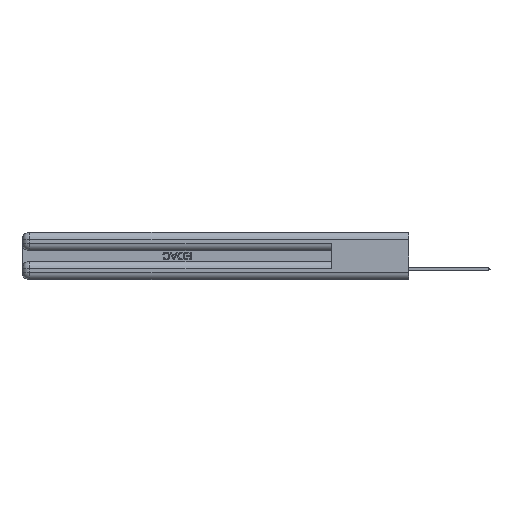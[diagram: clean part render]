
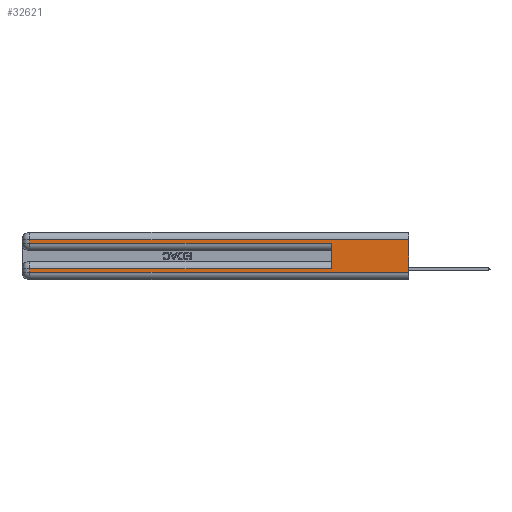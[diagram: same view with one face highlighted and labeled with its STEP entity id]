
A CAD part, left-side view. The second image highlights one B-rep face of the part: STEP entity #32621.
In plain terms, the highlighted planar face has unit normal (-1, 0, 0).
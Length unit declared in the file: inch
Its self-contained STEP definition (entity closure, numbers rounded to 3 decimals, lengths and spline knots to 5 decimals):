
#1006 = EDGE_CURVE ( 'NONE', #19458, #11600, #33406, .T. ) ;
#1236 = VECTOR ( 'NONE', #7126, 39.37008 ) ;
#3824 = CARTESIAN_POINT ( 'NONE',  ( 0., 0., 0.06 ) ) ;
#3852 = CARTESIAN_POINT ( 'NONE',  ( 0., 2.94, 0.06 ) ) ;
#3919 = VECTOR ( 'NONE', #11406, 39.37008 ) ;
#4619 = VECTOR ( 'NONE', #36373, 39.37008 ) ;
#5745 = VERTEX_POINT ( 'NONE', #46463 ) ;
#6093 = CARTESIAN_POINT ( 'NONE',  ( 0., 2.94, 0.31 ) ) ;
#6410 = LINE ( 'NONE', #38191, #3919 ) ;
#6543 = DIRECTION ( 'NONE',  ( 0., 1., 0. ) ) ;
#6690 = EDGE_CURVE ( 'NONE', #17661, #47163, #33459, .T. ) ;
#7126 = DIRECTION ( 'NONE',  ( 0., 1., 0. ) ) ;
#7585 = LINE ( 'NONE', #3824, #41613 ) ;
#8879 = CARTESIAN_POINT ( 'NONE',  ( 0., 2.94, 0.085 ) ) ;
#9315 = VERTEX_POINT ( 'NONE', #3852 ) ;
#9383 = ORIENTED_EDGE ( 'NONE', *, *, #12408, .T. ) ;
#11406 = DIRECTION ( 'NONE',  ( 0., -1., 0. ) ) ;
#11463 = CARTESIAN_POINT ( 'NONE',  ( 0., 0., 0.31 ) ) ;
#11600 = VERTEX_POINT ( 'NONE', #6093 ) ;
#12283 = ORIENTED_EDGE ( 'NONE', *, *, #15219, .T. ) ;
#12408 = EDGE_CURVE ( 'NONE', #11600, #37353, #27180, .T. ) ;
#15219 = EDGE_CURVE ( 'NONE', #9315, #5745, #7585, .T. ) ;
#16468 = LINE ( 'NONE', #27499, #38586 ) ;
#16790 = ORIENTED_EDGE ( 'NONE', *, *, #1006, .T. ) ;
#17089 = PLANE ( 'NONE',  #28386 ) ;
#17661 = VERTEX_POINT ( 'NONE', #50497 ) ;
#18962 = VECTOR ( 'NONE', #6543, 39.37008 ) ;
#19458 = VERTEX_POINT ( 'NONE', #26622 ) ;
#21163 = EDGE_CURVE ( 'NONE', #19458, #5745, #16468, .T. ) ;
#21610 = EDGE_CURVE ( 'NONE', #37353, #49317, #6410, .T. ) ;
#21665 = CARTESIAN_POINT ( 'NONE',  ( 0., 0., 0.37 ) ) ;
#22977 = ORIENTED_EDGE ( 'NONE', *, *, #21610, .T. ) ;
#23033 = DIRECTION ( 'NONE',  ( 0., 0., -1. ) ) ;
#24056 = EDGE_CURVE ( 'NONE', #17661, #49317, #38378, .T. ) ;
#25416 = DIRECTION ( 'NONE',  ( 0., 0., -1. ) ) ;
#26622 = CARTESIAN_POINT ( 'NONE',  ( 0., 0., 0.31 ) ) ;
#27152 = ORIENTED_EDGE ( 'NONE', *, *, #24056, .F. ) ;
#27180 = LINE ( 'NONE', #50384, #32761 ) ;
#27499 = CARTESIAN_POINT ( 'NONE',  ( 0., 0., 0.37 ) ) ;
#27632 = ORIENTED_EDGE ( 'NONE', *, *, #51509, .T. ) ;
#28237 = DIRECTION ( 'NONE',  ( 0., 0., 1. ) ) ;
#28386 = AXIS2_PLACEMENT_3D ( 'NONE', #21665, #29822, #25416 ) ;
#29822 = DIRECTION ( 'NONE',  ( 1., 0., 0. ) ) ;
#32025 = DIRECTION ( 'NONE',  ( 0., -1., 0. ) ) ;
#32104 = VECTOR ( 'NONE', #28237, 39.37008 ) ;
#32621 = ADVANCED_FACE ( 'NONE', ( #38972 ), #17089, .F. ) ;
#32761 = VECTOR ( 'NONE', #23033, 39.37008 ) ;
#33406 = LINE ( 'NONE', #11463, #1236 ) ;
#33459 = LINE ( 'NONE', #34942, #18962 ) ;
#34942 = CARTESIAN_POINT ( 'NONE',  ( 0., 0., 0.085 ) ) ;
#35229 = CARTESIAN_POINT ( 'NONE',  ( 0., 0.6, 0.285 ) ) ;
#36219 = CARTESIAN_POINT ( 'NONE',  ( 0., 2.94, 0.37 ) ) ;
#36373 = DIRECTION ( 'NONE',  ( 0., 0., -1. ) ) ;
#37353 = VERTEX_POINT ( 'NONE', #43759 ) ;
#37684 = ORIENTED_EDGE ( 'NONE', *, *, #21163, .F. ) ;
#38191 = CARTESIAN_POINT ( 'NONE',  ( 0., 0., 0.285 ) ) ;
#38378 = LINE ( 'NONE', #44173, #32104 ) ;
#38586 = VECTOR ( 'NONE', #39308, 39.37008 ) ;
#38972 = FACE_OUTER_BOUND ( 'NONE', #44858, .T. ) ;
#39308 = DIRECTION ( 'NONE',  ( 0., 0., -1. ) ) ;
#39989 = LINE ( 'NONE', #36219, #4619 ) ;
#41613 = VECTOR ( 'NONE', #32025, 39.37008 ) ;
#42167 = ORIENTED_EDGE ( 'NONE', *, *, #6690, .T. ) ;
#43759 = CARTESIAN_POINT ( 'NONE',  ( 0., 2.94, 0.285 ) ) ;
#44173 = CARTESIAN_POINT ( 'NONE',  ( 0., 0.6, 0.145 ) ) ;
#44858 = EDGE_LOOP ( 'NONE', ( #37684, #16790, #9383, #22977, #27152, #42167, #27632, #12283 ) ) ;
#46463 = CARTESIAN_POINT ( 'NONE',  ( 0., 0., 0.06 ) ) ;
#47163 = VERTEX_POINT ( 'NONE', #8879 ) ;
#49317 = VERTEX_POINT ( 'NONE', #35229 ) ;
#50384 = CARTESIAN_POINT ( 'NONE',  ( 0., 2.94, 0.37 ) ) ;
#50497 = CARTESIAN_POINT ( 'NONE',  ( 0., 0.6, 0.085 ) ) ;
#51509 = EDGE_CURVE ( 'NONE', #47163, #9315, #39989, .T. ) ;
